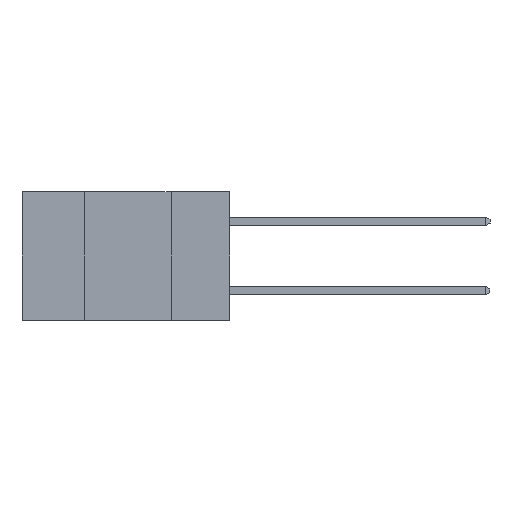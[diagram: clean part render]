
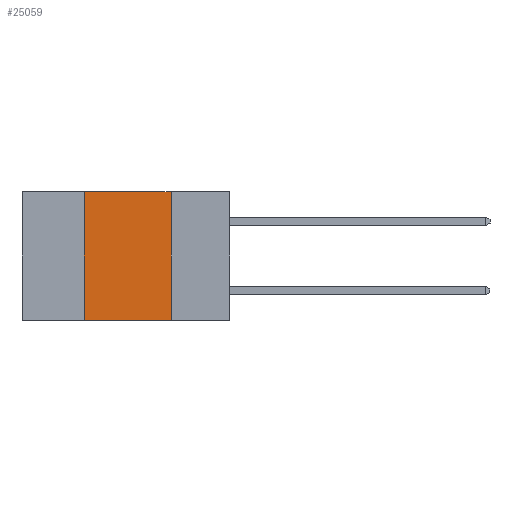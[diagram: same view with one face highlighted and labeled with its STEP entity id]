
A CAD part, left-side view. The second image highlights one B-rep face of the part: STEP entity #25059.
In plain terms, the highlighted planar face has unit normal (-1, 0, 0).
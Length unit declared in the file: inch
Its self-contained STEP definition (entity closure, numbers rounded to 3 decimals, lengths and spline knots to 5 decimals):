
#1073 = VECTOR ( 'NONE', #16826, 39.37008 ) ;
#1499 = CARTESIAN_POINT ( 'NONE',  ( 0., 0.42, 0. ) ) ;
#1583 = VERTEX_POINT ( 'NONE', #5446 ) ;
#2092 = ORIENTED_EDGE ( 'NONE', *, *, #16860, .F. ) ;
#2898 = DIRECTION ( 'NONE',  ( 0., 0., -1. ) ) ;
#4836 = EDGE_CURVE ( 'NONE', #13954, #1583, #15039, .T. ) ;
#4867 = CARTESIAN_POINT ( 'NONE',  ( 0., 0.17, 0. ) ) ;
#4961 = DIRECTION ( 'NONE',  ( 0., 0., -1. ) ) ;
#5161 = EDGE_CURVE ( 'NONE', #13954, #22159, #6604, .T. ) ;
#5179 = VECTOR ( 'NONE', #24921, 39.37008 ) ;
#5446 = CARTESIAN_POINT ( 'NONE',  ( 0., 0.42, 0. ) ) ;
#5828 = CARTESIAN_POINT ( 'NONE',  ( 0., 0.17, 0. ) ) ;
#6604 = LINE ( 'NONE', #7146, #5179 ) ;
#7146 = CARTESIAN_POINT ( 'NONE',  ( 0., 0.6, -0.37 ) ) ;
#8469 = VERTEX_POINT ( 'NONE', #5828 ) ;
#10649 = EDGE_CURVE ( 'NONE', #1583, #8469, #24730, .T. ) ;
#11821 = PLANE ( 'NONE',  #26268 ) ;
#11964 = ORIENTED_EDGE ( 'NONE', *, *, #4836, .F. ) ;
#12418 = ORIENTED_EDGE ( 'NONE', *, *, #5161, .T. ) ;
#13162 = LINE ( 'NONE', #4867, #24225 ) ;
#13954 = VERTEX_POINT ( 'NONE', #15309 ) ;
#14094 = CARTESIAN_POINT ( 'NONE',  ( 0., 0.6, 0. ) ) ;
#14357 = VECTOR ( 'NONE', #23898, 39.37008 ) ;
#14594 = CARTESIAN_POINT ( 'NONE',  ( 0., 0.6, 0. ) ) ;
#15039 = LINE ( 'NONE', #1499, #14357 ) ;
#15309 = CARTESIAN_POINT ( 'NONE',  ( 0., 0.42, -0.37 ) ) ;
#16319 = DIRECTION ( 'NONE',  ( 1., 0., 0. ) ) ;
#16826 = DIRECTION ( 'NONE',  ( 0., -1., 0. ) ) ;
#16860 = EDGE_CURVE ( 'NONE', #8469, #22159, #13162, .T. ) ;
#18091 = CARTESIAN_POINT ( 'NONE',  ( 0., 0.17, -0.37 ) ) ;
#20040 = EDGE_LOOP ( 'NONE', ( #2092, #20795, #11964, #12418 ) ) ;
#20795 = ORIENTED_EDGE ( 'NONE', *, *, #10649, .F. ) ;
#22159 = VERTEX_POINT ( 'NONE', #18091 ) ;
#23898 = DIRECTION ( 'NONE',  ( 0., 0., 1. ) ) ;
#24225 = VECTOR ( 'NONE', #4961, 39.37008 ) ;
#24730 = LINE ( 'NONE', #14594, #1073 ) ;
#24921 = DIRECTION ( 'NONE',  ( 0., -1., 0. ) ) ;
#25059 = ADVANCED_FACE ( 'NONE', ( #26718 ), #11821, .F. ) ;
#26268 = AXIS2_PLACEMENT_3D ( 'NONE', #14094, #16319, #2898 ) ;
#26718 = FACE_OUTER_BOUND ( 'NONE', #20040, .T. ) ;
